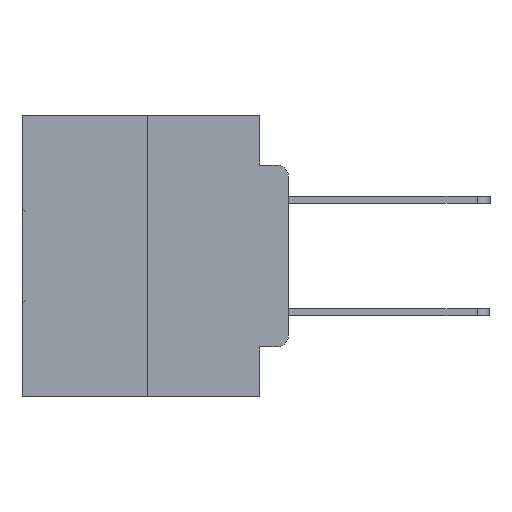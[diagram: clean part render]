
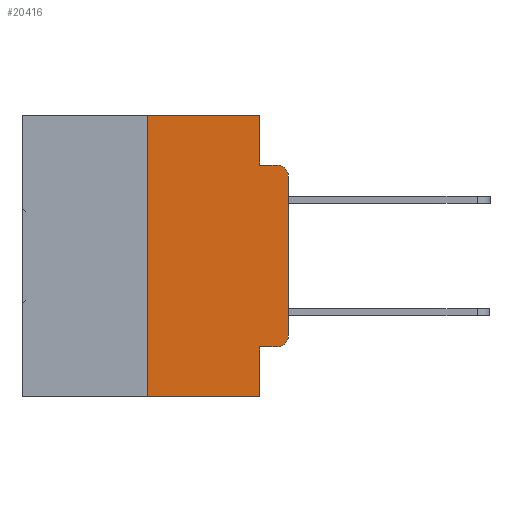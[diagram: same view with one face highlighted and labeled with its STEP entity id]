
A CAD part, left-side view. The second image highlights one B-rep face of the part: STEP entity #20416.
In plain terms, the highlighted planar face has unit normal (-1, 0, 0).
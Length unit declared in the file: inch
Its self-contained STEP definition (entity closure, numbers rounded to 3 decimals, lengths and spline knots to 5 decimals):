
#795 = CARTESIAN_POINT ( 'NONE',  ( 0., 0.25, 0. ) ) ;
#1514 = EDGE_CURVE ( 'NONE', #12836, #33243, #32166, .T. ) ;
#1562 = EDGE_CURVE ( 'NONE', #12836, #10929, #3086, .T. ) ;
#1674 = CARTESIAN_POINT ( 'NONE',  ( 0., 0.051, -0.4115 ) ) ;
#2434 = CARTESIAN_POINT ( 'NONE',  ( 0., 0.25, 0. ) ) ;
#2609 = FACE_OUTER_BOUND ( 'NONE', #20165, .T. ) ;
#3086 = LINE ( 'NONE', #1674, #3893 ) ;
#3238 = CARTESIAN_POINT ( 'NONE',  ( 0., 0.473, 0. ) ) ;
#3522 = AXIS2_PLACEMENT_3D ( 'NONE', #8491, #26616, #11090 ) ;
#3825 = CARTESIAN_POINT ( 'NONE',  ( 0., 0.051, -0.4115 ) ) ;
#3893 = VECTOR ( 'NONE', #30748, 39.37008 ) ;
#3906 = ORIENTED_EDGE ( 'NONE', *, *, #6677, .F. ) ;
#4165 = CARTESIAN_POINT ( 'NONE',  ( 0., 0.473, -0.5 ) ) ;
#4589 = CARTESIAN_POINT ( 'NONE',  ( 0., 0.25, -0.5 ) ) ;
#4657 = VERTEX_POINT ( 'NONE', #21291 ) ;
#5005 = ORIENTED_EDGE ( 'NONE', *, *, #1562, .T. ) ;
#5545 = VERTEX_POINT ( 'NONE', #11549 ) ;
#6013 = LINE ( 'NONE', #795, #32660 ) ;
#6677 = EDGE_CURVE ( 'NONE', #7689, #14557, #6013, .T. ) ;
#7196 = ORIENTED_EDGE ( 'NONE', *, *, #11107, .T. ) ;
#7535 = VECTOR ( 'NONE', #24051, 39.37008 ) ;
#7689 = VERTEX_POINT ( 'NONE', #4589 ) ;
#8491 = CARTESIAN_POINT ( 'NONE',  ( 0., 0.02, -0.3915 ) ) ;
#9045 = ORIENTED_EDGE ( 'NONE', *, *, #1514, .F. ) ;
#9388 = DIRECTION ( 'NONE',  ( 0., -1., 0. ) ) ;
#10159 = CARTESIAN_POINT ( 'NONE',  ( 0., 0.02, -0.1085 ) ) ;
#10247 = ORIENTED_EDGE ( 'NONE', *, *, #15662, .T. ) ;
#10335 = ORIENTED_EDGE ( 'NONE', *, *, #23580, .F. ) ;
#10551 = CARTESIAN_POINT ( 'NONE',  ( 0., 0.473, 0. ) ) ;
#10677 = EDGE_CURVE ( 'NONE', #5545, #26088, #12843, .T. ) ;
#10929 = VERTEX_POINT ( 'NONE', #27503 ) ;
#11047 = PLANE ( 'NONE',  #29489 ) ;
#11090 = DIRECTION ( 'NONE',  ( 0., 0., -1. ) ) ;
#11107 = EDGE_CURVE ( 'NONE', #30180, #26088, #22182, .T. ) ;
#11549 = CARTESIAN_POINT ( 'NONE',  ( 0., 0.051, -0.0885 ) ) ;
#12232 = CARTESIAN_POINT ( 'NONE',  ( 0., 0.051, 0. ) ) ;
#12713 = EDGE_CURVE ( 'NONE', #10929, #4657, #32034, .T. ) ;
#12797 = DIRECTION ( 'NONE',  ( 0., 0., -1. ) ) ;
#12836 = VERTEX_POINT ( 'NONE', #3825 ) ;
#12843 = LINE ( 'NONE', #16359, #7535 ) ;
#12946 = EDGE_CURVE ( 'NONE', #7689, #33243, #31623, .T. ) ;
#12950 = LINE ( 'NONE', #32674, #19078 ) ;
#13457 = ORIENTED_EDGE ( 'NONE', *, *, #23830, .F. ) ;
#13687 = DIRECTION ( 'NONE',  ( 0., 0., -1. ) ) ;
#14523 = CARTESIAN_POINT ( 'NONE',  ( 0., 0., 0. ) ) ;
#14557 = VERTEX_POINT ( 'NONE', #2434 ) ;
#14766 = DIRECTION ( 'NONE',  ( 0., 0., -1. ) ) ;
#15662 = EDGE_CURVE ( 'NONE', #4657, #30180, #30450, .T. ) ;
#16359 = CARTESIAN_POINT ( 'NONE',  ( 0., 0.051, -0.0885 ) ) ;
#18658 = VECTOR ( 'NONE', #26068, 39.37008 ) ;
#18980 = AXIS2_PLACEMENT_3D ( 'NONE', #10159, #28260, #12797 ) ;
#19078 = VECTOR ( 'NONE', #25099, 39.37008 ) ;
#20165 = EDGE_LOOP ( 'NONE', ( #10247, #7196, #29321, #10335, #13457, #3906, #25384, #9045, #5005, #24419 ) ) ;
#20416 = ADVANCED_FACE ( 'NONE', ( #2609 ), #11047, .F. ) ;
#20872 = VERTEX_POINT ( 'NONE', #25745 ) ;
#21291 = CARTESIAN_POINT ( 'NONE',  ( 0., 0., -0.3915 ) ) ;
#22182 = CIRCLE ( 'NONE', #18980, 0.02 ) ;
#23209 = CARTESIAN_POINT ( 'NONE',  ( 0., 0.02, -0.0885 ) ) ;
#23580 = EDGE_CURVE ( 'NONE', #20872, #5545, #12950, .T. ) ;
#23669 = VECTOR ( 'NONE', #24929, 39.37008 ) ;
#23830 = EDGE_CURVE ( 'NONE', #14557, #20872, #32260, .T. ) ;
#24051 = DIRECTION ( 'NONE',  ( 0., -1., 0. ) ) ;
#24143 = CARTESIAN_POINT ( 'NONE',  ( 0., 0., -0.1085 ) ) ;
#24192 = DIRECTION ( 'NONE',  ( 0., 0., 1. ) ) ;
#24419 = ORIENTED_EDGE ( 'NONE', *, *, #12713, .T. ) ;
#24420 = CARTESIAN_POINT ( 'NONE',  ( 0., 0.051, -0.5 ) ) ;
#24837 = VECTOR ( 'NONE', #9388, 39.37008 ) ;
#24929 = DIRECTION ( 'NONE',  ( 0., 0., 1. ) ) ;
#25099 = DIRECTION ( 'NONE',  ( 0., 0., -1. ) ) ;
#25384 = ORIENTED_EDGE ( 'NONE', *, *, #12946, .T. ) ;
#25745 = CARTESIAN_POINT ( 'NONE',  ( 0., 0.051, 0. ) ) ;
#26068 = DIRECTION ( 'NONE',  ( 0., -1., 0. ) ) ;
#26088 = VERTEX_POINT ( 'NONE', #23209 ) ;
#26616 = DIRECTION ( 'NONE',  ( -1., 0., 0. ) ) ;
#27503 = CARTESIAN_POINT ( 'NONE',  ( 0., 0.02, -0.4115 ) ) ;
#28260 = DIRECTION ( 'NONE',  ( -1., 0., 0. ) ) ;
#29136 = DIRECTION ( 'NONE',  ( 1., 0., 0. ) ) ;
#29321 = ORIENTED_EDGE ( 'NONE', *, *, #10677, .F. ) ;
#29489 = AXIS2_PLACEMENT_3D ( 'NONE', #3238, #29136, #13687 ) ;
#30180 = VERTEX_POINT ( 'NONE', #24143 ) ;
#30450 = LINE ( 'NONE', #14523, #23669 ) ;
#30748 = DIRECTION ( 'NONE',  ( 0., -1., 0. ) ) ;
#31367 = VECTOR ( 'NONE', #14766, 39.37008 ) ;
#31623 = LINE ( 'NONE', #4165, #24837 ) ;
#32034 = CIRCLE ( 'NONE', #3522, 0.02 ) ;
#32166 = LINE ( 'NONE', #12232, #31367 ) ;
#32260 = LINE ( 'NONE', #10551, #18658 ) ;
#32660 = VECTOR ( 'NONE', #24192, 39.37008 ) ;
#32674 = CARTESIAN_POINT ( 'NONE',  ( 0., 0.051, 0. ) ) ;
#33243 = VERTEX_POINT ( 'NONE', #24420 ) ;
